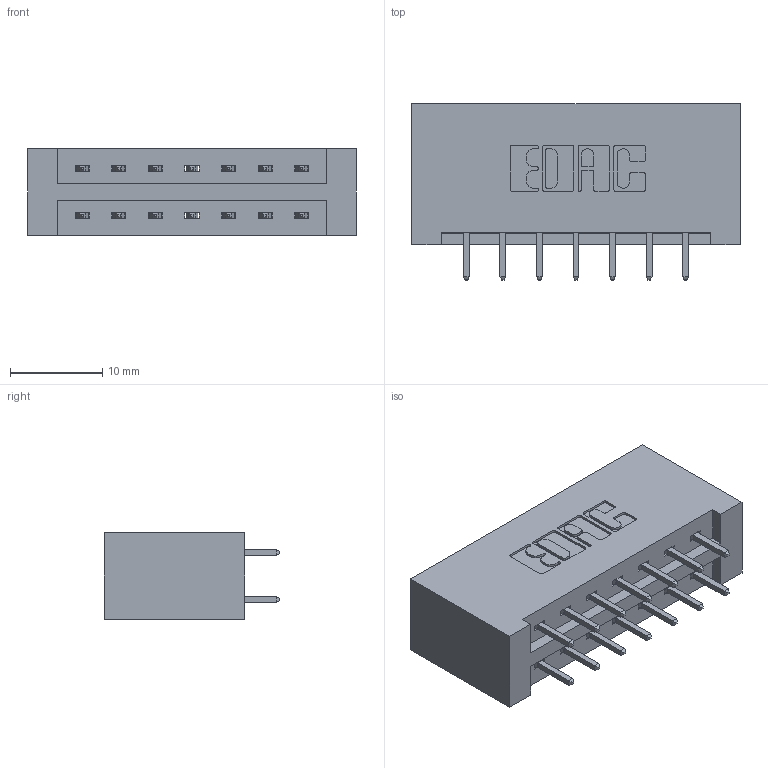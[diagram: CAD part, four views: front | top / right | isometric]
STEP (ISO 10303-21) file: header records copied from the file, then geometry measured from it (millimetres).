
FILE_DESCRIPTION (( 'STEP AP203' ), '1' );
FILE_NAME ('337-014-521-201.STEP', '2018-08-04T14:02:59', ( '' ), ( '' ), 'SwSTEP 2.0', 'SolidWorks 2016', '' );
FILE_SCHEMA (( 'CONFIG_CONTROL_DESIGN' ));
Length unit declared in the file: inch
Products named in the file (3): 345-292-001_345-293-121; 337-014-521-201; 337 Part_No Mounting Lugs
Assembly tree (15 placements, depth 2):
  337-014-521-201
    337 Part_No Mounting Lugs
    345-292-001_345-293-121  x14
Bounding box: 35.61 x 19.06 x 9.4 mm (x, y, z)
Volume: 4042.1 mm3; surface area: 4244.2 mm2
Topology: 15 solids, 15 shells, 862 faces, 2541 edges, 1674 vertices
Faces by surface type: plane 598, cylinder 264
Entity records: 9695 total; most frequent: CARTESIAN_POINT 1662, ORIENTED_EDGE 1598, DIRECTION 1471, EDGE_CURVE 799, VECTOR 679, LINE 679, VERTEX_POINT 530, AXIS2_PLACEMENT_3D 396
